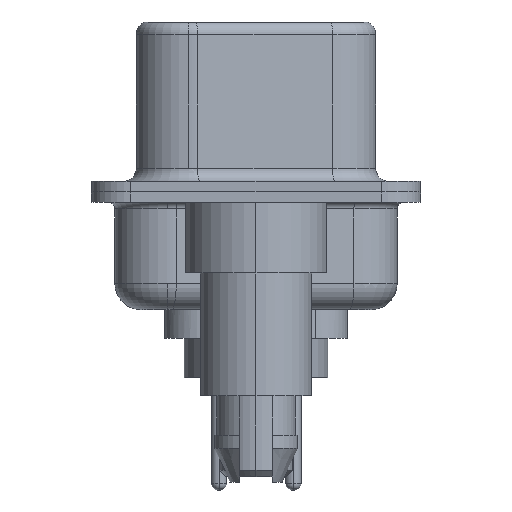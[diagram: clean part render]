
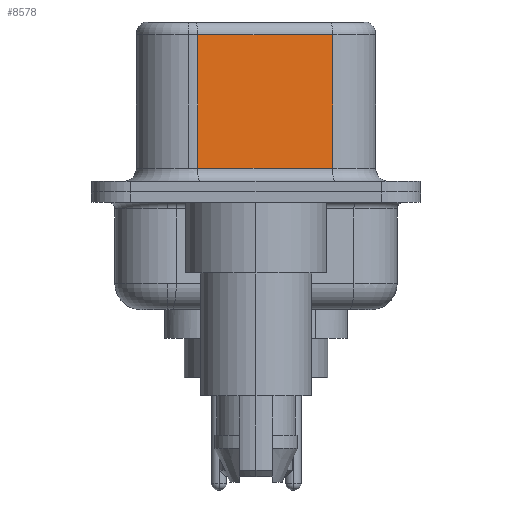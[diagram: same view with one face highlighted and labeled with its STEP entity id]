
A CAD part, left-side view. The second image highlights one B-rep face of the part: STEP entity #8578.
In plain terms, the highlighted planar face has unit normal (-0.985, -0.174, 0).
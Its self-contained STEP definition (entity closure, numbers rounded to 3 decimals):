
#63 = CARTESIAN_POINT ( 'NONE',  ( 4.565, -2.927, 6.52 ) ) ;
#119 = CARTESIAN_POINT ( 'NONE',  ( 4.565, -2.927, 0.9 ) ) ;
#581 = DIRECTION ( 'NONE',  ( 0., 0., -1. ) ) ;
#584 = AXIS2_PLACEMENT_3D ( 'NONE', #63, #5104, #14097 ) ;
#1336 = EDGE_CURVE ( 'NONE', #2469, #5015, #16477, .T. ) ;
#1418 = VERTEX_POINT ( 'NONE', #4486 ) ;
#2376 = DIRECTION ( 'NONE',  ( 0.174, -0.985, 0. ) ) ;
#2469 = VERTEX_POINT ( 'NONE', #3805 ) ;
#2512 = CARTESIAN_POINT ( 'NONE',  ( 3.655, 2.233, 6.52 ) ) ;
#3352 = CARTESIAN_POINT ( 'NONE',  ( 4.565, -2.927, 0.9 ) ) ;
#3644 = EDGE_CURVE ( 'NONE', #7095, #2469, #15572, .T. ) ;
#3805 = CARTESIAN_POINT ( 'NONE',  ( 3.655, 2.233, 0.9 ) ) ;
#3851 = PLANE ( 'NONE',  #584 ) ;
#4063 = CARTESIAN_POINT ( 'NONE',  ( 4.565, -2.927, 6.52 ) ) ;
#4110 = DIRECTION ( 'NONE',  ( 0., 0., -1. ) ) ;
#4486 = CARTESIAN_POINT ( 'NONE',  ( 4.565, -2.927, 6.02 ) ) ;
#5015 = VERTEX_POINT ( 'NONE', #119 ) ;
#5104 = DIRECTION ( 'NONE',  ( 0.985, 0.174, 0. ) ) ;
#5699 = VECTOR ( 'NONE', #581, 1000. ) ;
#5914 = VECTOR ( 'NONE', #4110, 1000. ) ;
#7095 = VERTEX_POINT ( 'NONE', #16064 ) ;
#8578 = ADVANCED_FACE ( 'NONE', ( #13726 ), #3851, .F. ) ;
#8821 = DIRECTION ( 'NONE',  ( -0.174, 0.985, 0. ) ) ;
#9624 = VECTOR ( 'NONE', #2376, 1000. ) ;
#10150 = CARTESIAN_POINT ( 'NONE',  ( 4.565, -2.927, 6.02 ) ) ;
#10395 = VECTOR ( 'NONE', #8821, 1000. ) ;
#10797 = LINE ( 'NONE', #10150, #10395 ) ;
#12375 = ORIENTED_EDGE ( 'NONE', *, *, #15110, .F. ) ;
#13616 = LINE ( 'NONE', #4063, #5914 ) ;
#13637 = EDGE_CURVE ( 'NONE', #1418, #7095, #10797, .T. ) ;
#13665 = ORIENTED_EDGE ( 'NONE', *, *, #1336, .T. ) ;
#13708 = ORIENTED_EDGE ( 'NONE', *, *, #13637, .T. ) ;
#13726 = FACE_OUTER_BOUND ( 'NONE', #15612, .T. ) ;
#14097 = DIRECTION ( 'NONE',  ( -0.174, 0.985, 0. ) ) ;
#14269 = ORIENTED_EDGE ( 'NONE', *, *, #3644, .T. ) ;
#15110 = EDGE_CURVE ( 'NONE', #1418, #5015, #13616, .T. ) ;
#15572 = LINE ( 'NONE', #2512, #5699 ) ;
#15612 = EDGE_LOOP ( 'NONE', ( #12375, #13708, #14269, #13665 ) ) ;
#16064 = CARTESIAN_POINT ( 'NONE',  ( 3.655, 2.233, 6.02 ) ) ;
#16477 = LINE ( 'NONE', #3352, #9624 ) ;
